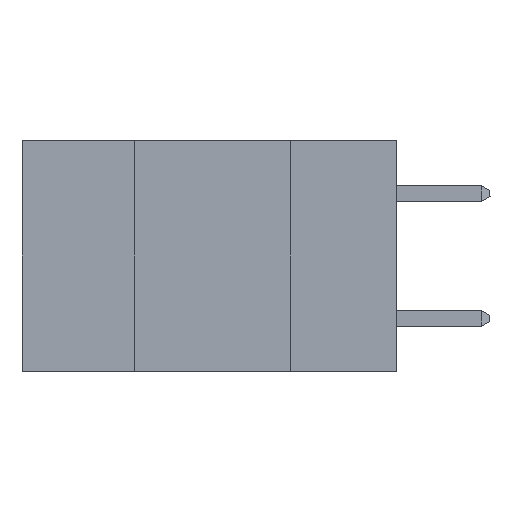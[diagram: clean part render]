
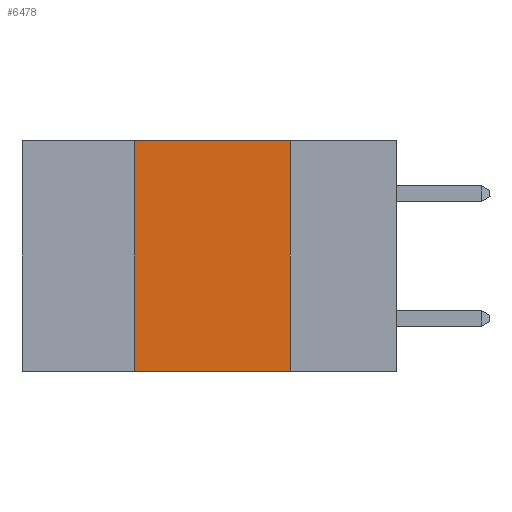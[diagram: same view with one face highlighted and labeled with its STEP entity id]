
A CAD part, left-side view. The second image highlights one B-rep face of the part: STEP entity #6478.
In plain terms, the highlighted planar face has unit normal (-1, 0, 0).
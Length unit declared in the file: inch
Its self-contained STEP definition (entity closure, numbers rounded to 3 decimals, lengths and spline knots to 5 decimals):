
#112 = VERTEX_POINT ( 'NONE', #4697 ) ;
#573 = ORIENTED_EDGE ( 'NONE', *, *, #12881, .F. ) ;
#1071 = VECTOR ( 'NONE', #9262, 39.37008 ) ;
#1215 = LINE ( 'NONE', #7934, #13504 ) ;
#1753 = LINE ( 'NONE', #5417, #14591 ) ;
#2311 = ORIENTED_EDGE ( 'NONE', *, *, #9577, .T. ) ;
#2322 = EDGE_CURVE ( 'NONE', #2374, #2531, #1215, .T. ) ;
#2374 = VERTEX_POINT ( 'NONE', #14038 ) ;
#2531 = VERTEX_POINT ( 'NONE', #15866 ) ;
#2740 = VERTEX_POINT ( 'NONE', #3732 ) ;
#3095 = EDGE_LOOP ( 'NONE', ( #3415, #11916, #573, #2311 ) ) ;
#3415 = ORIENTED_EDGE ( 'NONE', *, *, #4929, .F. ) ;
#3732 = CARTESIAN_POINT ( 'NONE',  ( 0., 0.42, -0.37 ) ) ;
#4261 = LINE ( 'NONE', #7342, #9799 ) ;
#4280 = CARTESIAN_POINT ( 'NONE',  ( 0., 0.42, 0. ) ) ;
#4697 = CARTESIAN_POINT ( 'NONE',  ( 0., 0.17, -0.37 ) ) ;
#4929 = EDGE_CURVE ( 'NONE', #2531, #112, #4261, .T. ) ;
#5417 = CARTESIAN_POINT ( 'NONE',  ( 0., 0.6, -0.37 ) ) ;
#6478 = ADVANCED_FACE ( 'NONE', ( #12791 ), #11185, .F. ) ;
#6668 = LINE ( 'NONE', #4280, #1071 ) ;
#7342 = CARTESIAN_POINT ( 'NONE',  ( 0., 0.17, 0. ) ) ;
#7441 = DIRECTION ( 'NONE',  ( 0., 0., -1. ) ) ;
#7934 = CARTESIAN_POINT ( 'NONE',  ( 0., 0.6, 0. ) ) ;
#9262 = DIRECTION ( 'NONE',  ( 0., 0., 1. ) ) ;
#9577 = EDGE_CURVE ( 'NONE', #2740, #112, #1753, .T. ) ;
#9799 = VECTOR ( 'NONE', #12454, 39.37008 ) ;
#11185 = PLANE ( 'NONE',  #13595 ) ;
#11507 = DIRECTION ( 'NONE',  ( 0., -1., 0. ) ) ;
#11916 = ORIENTED_EDGE ( 'NONE', *, *, #2322, .F. ) ;
#12397 = CARTESIAN_POINT ( 'NONE',  ( 0., 0.6, 0. ) ) ;
#12454 = DIRECTION ( 'NONE',  ( 0., 0., -1. ) ) ;
#12791 = FACE_OUTER_BOUND ( 'NONE', #3095, .T. ) ;
#12881 = EDGE_CURVE ( 'NONE', #2740, #2374, #6668, .T. ) ;
#13504 = VECTOR ( 'NONE', #11507, 39.37008 ) ;
#13548 = DIRECTION ( 'NONE',  ( 1., 0., 0. ) ) ;
#13595 = AXIS2_PLACEMENT_3D ( 'NONE', #12397, #13548, #7441 ) ;
#14038 = CARTESIAN_POINT ( 'NONE',  ( 0., 0.42, 0. ) ) ;
#14591 = VECTOR ( 'NONE', #15239, 39.37008 ) ;
#15239 = DIRECTION ( 'NONE',  ( 0., -1., 0. ) ) ;
#15866 = CARTESIAN_POINT ( 'NONE',  ( 0., 0.17, 0. ) ) ;
